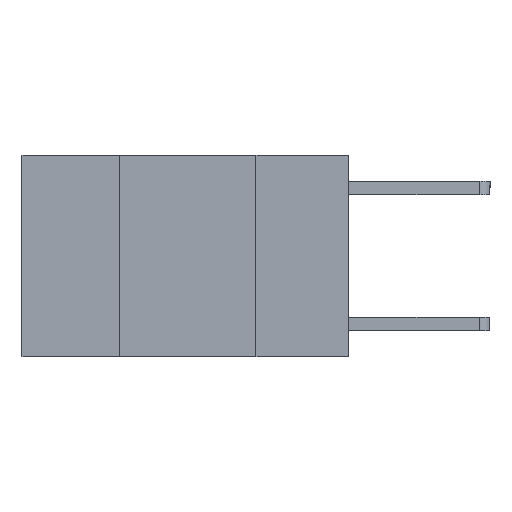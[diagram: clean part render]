
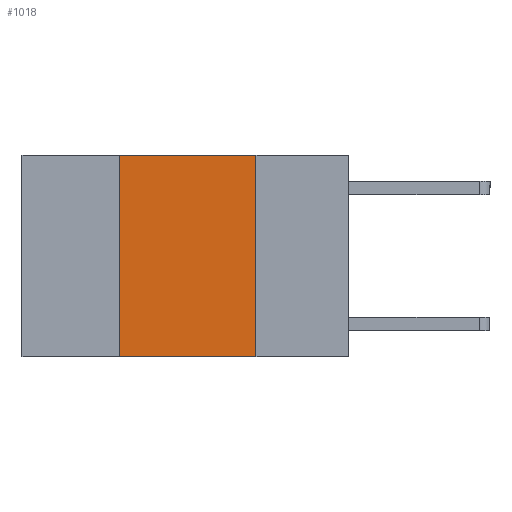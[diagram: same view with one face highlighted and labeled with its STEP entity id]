
A CAD part, left-side view. The second image highlights one B-rep face of the part: STEP entity #1018.
In plain terms, the highlighted planar face has unit normal (-1, 0, 0).
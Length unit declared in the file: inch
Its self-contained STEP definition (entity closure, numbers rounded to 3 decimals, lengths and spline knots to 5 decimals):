
#24 = PLANE ( 'NONE',  #1296 ) ;
#478 = LINE ( 'NONE', #8521, #4957 ) ;
#706 = VECTOR ( 'NONE', #8237, 39.37008 ) ;
#760 = CARTESIAN_POINT ( 'NONE',  ( 0., 0.17, 0. ) ) ;
#1018 = ADVANCED_FACE ( 'NONE', ( #5591 ), #24, .F. ) ;
#1036 = CARTESIAN_POINT ( 'NONE',  ( 0., 0.42, 0. ) ) ;
#1296 = AXIS2_PLACEMENT_3D ( 'NONE', #1674, #2551, #8805 ) ;
#1320 = DIRECTION ( 'NONE',  ( 0., 0., 1. ) ) ;
#1674 = CARTESIAN_POINT ( 'NONE',  ( 0., 0.6, 0. ) ) ;
#1881 = CARTESIAN_POINT ( 'NONE',  ( 0., 0.42, -0.37 ) ) ;
#2219 = VERTEX_POINT ( 'NONE', #8544 ) ;
#2551 = DIRECTION ( 'NONE',  ( 1., 0., 0. ) ) ;
#3348 = CARTESIAN_POINT ( 'NONE',  ( 0., 0.17, 0. ) ) ;
#3787 = EDGE_CURVE ( 'NONE', #8411, #2219, #4138, .T. ) ;
#4138 = LINE ( 'NONE', #3348, #9639 ) ;
#4330 = ORIENTED_EDGE ( 'NONE', *, *, #6323, .T. ) ;
#4351 = VECTOR ( 'NONE', #10237, 39.37008 ) ;
#4466 = EDGE_CURVE ( 'NONE', #6363, #8411, #7643, .T. ) ;
#4590 = CARTESIAN_POINT ( 'NONE',  ( 0., 0.6, 0. ) ) ;
#4957 = VECTOR ( 'NONE', #1320, 39.37008 ) ;
#5465 = EDGE_LOOP ( 'NONE', ( #10167, #10357, #5503, #4330 ) ) ;
#5503 = ORIENTED_EDGE ( 'NONE', *, *, #6849, .F. ) ;
#5591 = FACE_OUTER_BOUND ( 'NONE', #5465, .T. ) ;
#5921 = CARTESIAN_POINT ( 'NONE',  ( 0., 0.6, -0.37 ) ) ;
#6323 = EDGE_CURVE ( 'NONE', #6394, #2219, #9973, .T. ) ;
#6363 = VERTEX_POINT ( 'NONE', #1036 ) ;
#6394 = VERTEX_POINT ( 'NONE', #1881 ) ;
#6849 = EDGE_CURVE ( 'NONE', #6394, #6363, #478, .T. ) ;
#7258 = DIRECTION ( 'NONE',  ( 0., 0., -1. ) ) ;
#7643 = LINE ( 'NONE', #4590, #4351 ) ;
#8237 = DIRECTION ( 'NONE',  ( 0., -1., 0. ) ) ;
#8411 = VERTEX_POINT ( 'NONE', #760 ) ;
#8521 = CARTESIAN_POINT ( 'NONE',  ( 0., 0.42, 0. ) ) ;
#8544 = CARTESIAN_POINT ( 'NONE',  ( 0., 0.17, -0.37 ) ) ;
#8805 = DIRECTION ( 'NONE',  ( 0., 0., -1. ) ) ;
#9639 = VECTOR ( 'NONE', #7258, 39.37008 ) ;
#9973 = LINE ( 'NONE', #5921, #706 ) ;
#10167 = ORIENTED_EDGE ( 'NONE', *, *, #3787, .F. ) ;
#10237 = DIRECTION ( 'NONE',  ( 0., -1., 0. ) ) ;
#10357 = ORIENTED_EDGE ( 'NONE', *, *, #4466, .F. ) ;
